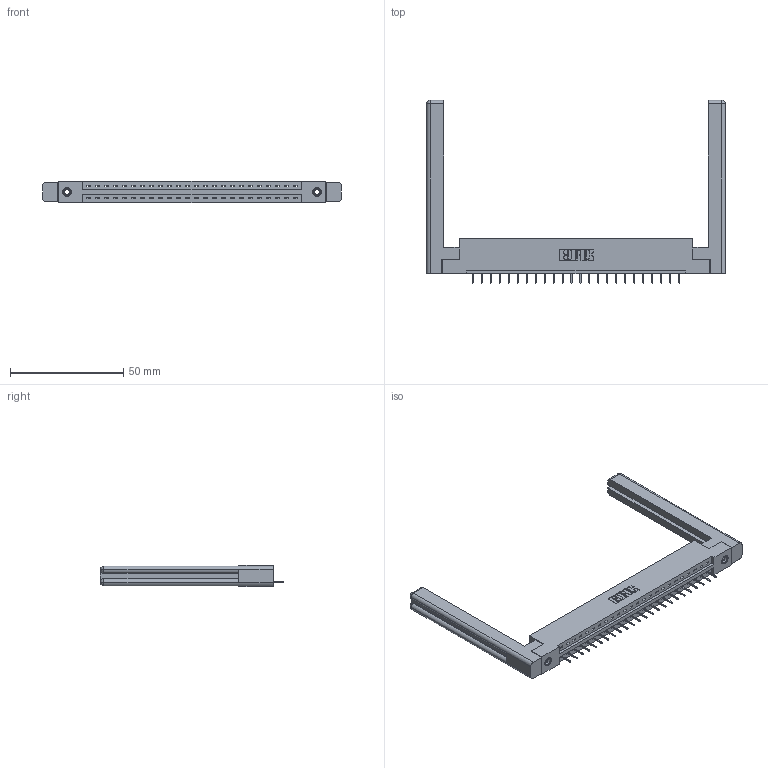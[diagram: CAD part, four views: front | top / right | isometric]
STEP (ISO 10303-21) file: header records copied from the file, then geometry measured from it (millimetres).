
FILE_DESCRIPTION (( 'STEP AP203' ), '1' );
FILE_NAME ('387-024-524-158.STEP', '2019-10-03T10:38:52', ( '' ), ( '' ), 'SwSTEP 2.0', 'SolidWorks 2016', '' );
FILE_SCHEMA (( 'CONFIG_CONTROL_DESIGN' ));
Length unit declared in the file: inch
Products named in the file (5): 387-024-524-158; 345-250-001_345-250-001-102; 307-220-058; 345-292-001_345-293-124; 337 Part_Flush Mounting Lugs - 0.156 Dia-TI
Assembly tree (29 placements, depth 2):
  387-024-524-158
    337 Part_Flush Mounting Lugs - 0.156 Dia-TI
    345-292-001_345-293-124  x24
    345-250-001_345-250-001-102  x2
    307-220-058  x2
Bounding box: 131.72 x 80.78 x 9.4 mm (x, y, z)
Volume: 20532.6 mm3; surface area: 18596.1 mm2
Topology: 29 solids, 29 shells, 1840 faces, 5273 edges, 3406 vertices
Faces by surface type: plane 1402, cylinder 414, cone 12, torus 12
Entity records: 22876 total; most frequent: CARTESIAN_POINT 3981, ORIENTED_EDGE 3880, DIRECTION 3408, EDGE_CURVE 1940, VECTOR 1768, LINE 1768, VERTEX_POINT 1282, AXIS2_PLACEMENT_3D 820
